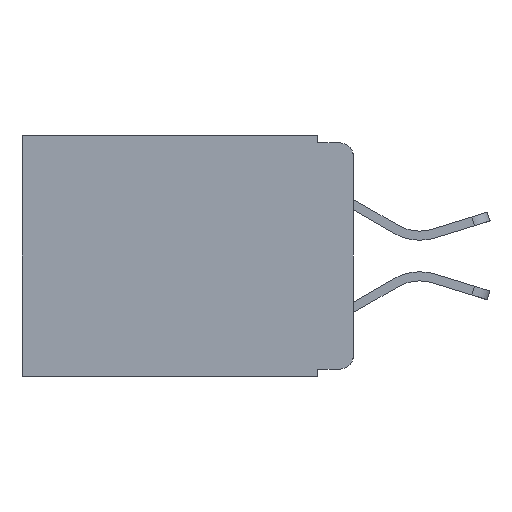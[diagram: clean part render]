
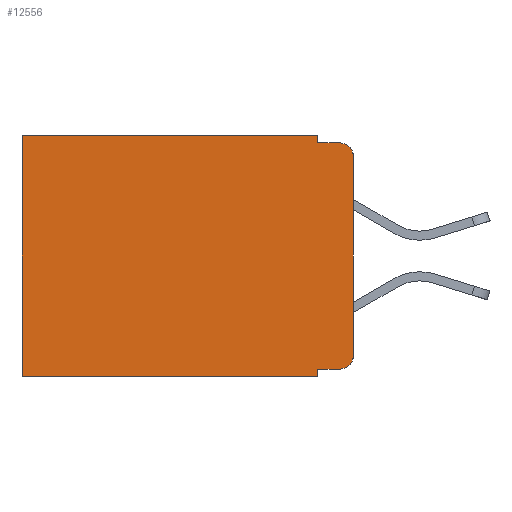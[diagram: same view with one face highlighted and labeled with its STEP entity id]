
A CAD part, left-side view. The second image highlights one B-rep face of the part: STEP entity #12556.
In plain terms, the highlighted planar face has unit normal (-1, 0, 0).
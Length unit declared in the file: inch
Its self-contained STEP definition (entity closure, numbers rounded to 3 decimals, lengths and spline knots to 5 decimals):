
#97 = EDGE_CURVE ( 'NONE', #14052, #8095, #5089, .T. ) ;
#119 = AXIS2_PLACEMENT_3D ( 'NONE', #12632, #4938, #13936 ) ;
#271 = CARTESIAN_POINT ( 'NONE',  ( 0.298, 0., 0. ) ) ;
#314 = CARTESIAN_POINT ( 'NONE',  ( 0.298, 0.051, -0.01 ) ) ;
#788 = ORIENTED_EDGE ( 'NONE', *, *, #12742, .T. ) ;
#1022 = CARTESIAN_POINT ( 'NONE',  ( 0.298, 0.02, -0.03 ) ) ;
#1136 = LINE ( 'NONE', #6046, #13415 ) ;
#1332 = CARTESIAN_POINT ( 'NONE',  ( 0.298, 0.051, 0. ) ) ;
#1670 = CARTESIAN_POINT ( 'NONE',  ( 0.298, 0.02, -0.333 ) ) ;
#1700 = FACE_OUTER_BOUND ( 'NONE', #5446, .T. ) ;
#1911 = VECTOR ( 'NONE', #9954, 39.37008 ) ;
#1912 = EDGE_CURVE ( 'NONE', #10570, #8095, #8886, .T. ) ;
#2055 = ORIENTED_EDGE ( 'NONE', *, *, #13623, .F. ) ;
#2117 = VERTEX_POINT ( 'NONE', #11443 ) ;
#2303 = VECTOR ( 'NONE', #10641, 39.37008 ) ;
#2398 = LINE ( 'NONE', #13743, #15792 ) ;
#2770 = VERTEX_POINT ( 'NONE', #1670 ) ;
#3006 = DIRECTION ( 'NONE',  ( 0., 0., -1. ) ) ;
#3040 = DIRECTION ( 'NONE',  ( -1., 0., 0. ) ) ;
#3200 = EDGE_CURVE ( 'NONE', #10178, #6726, #1136, .T. ) ;
#3749 = LINE ( 'NONE', #7935, #13255 ) ;
#4411 = CARTESIAN_POINT ( 'NONE',  ( 0.298, 0.051, -0.333 ) ) ;
#4774 = CIRCLE ( 'NONE', #119, 0.02 ) ;
#4907 = CARTESIAN_POINT ( 'NONE',  ( 0.298, 0.02, -0.01 ) ) ;
#4938 = DIRECTION ( 'NONE',  ( -1., 0., 0. ) ) ;
#4965 = VERTEX_POINT ( 'NONE', #5046 ) ;
#5046 = CARTESIAN_POINT ( 'NONE',  ( 0.298, 0., -0.313 ) ) ;
#5089 = LINE ( 'NONE', #314, #8149 ) ;
#5101 = CARTESIAN_POINT ( 'NONE',  ( 0.298, 0.051, -0.01 ) ) ;
#5204 = VECTOR ( 'NONE', #7310, 39.37008 ) ;
#5446 = EDGE_LOOP ( 'NONE', ( #7200, #6386, #6957, #6941, #7056, #12073, #5728, #2055, #788, #9640 ) ) ;
#5728 = ORIENTED_EDGE ( 'NONE', *, *, #10323, .F. ) ;
#5920 = LINE ( 'NONE', #6107, #1911 ) ;
#6046 = CARTESIAN_POINT ( 'NONE',  ( 0.298, 0., 0. ) ) ;
#6107 = CARTESIAN_POINT ( 'NONE',  ( 0.298, 0.051, -0.333 ) ) ;
#6386 = ORIENTED_EDGE ( 'NONE', *, *, #1912, .T. ) ;
#6726 = VERTEX_POINT ( 'NONE', #9935 ) ;
#6941 = ORIENTED_EDGE ( 'NONE', *, *, #16142, .F. ) ;
#6957 = ORIENTED_EDGE ( 'NONE', *, *, #97, .F. ) ;
#7056 = ORIENTED_EDGE ( 'NONE', *, *, #3200, .T. ) ;
#7086 = CARTESIAN_POINT ( 'NONE',  ( 0.298, 0.051, 0. ) ) ;
#7183 = VERTEX_POINT ( 'NONE', #4411 ) ;
#7200 = ORIENTED_EDGE ( 'NONE', *, *, #8176, .F. ) ;
#7310 = DIRECTION ( 'NONE',  ( 0., 0., -1. ) ) ;
#7895 = DIRECTION ( 'NONE',  ( 0., 0., -1. ) ) ;
#7935 = CARTESIAN_POINT ( 'NONE',  ( 0.298, 0., 0. ) ) ;
#8095 = VERTEX_POINT ( 'NONE', #4907 ) ;
#8149 = VECTOR ( 'NONE', #14157, 39.37008 ) ;
#8176 = EDGE_CURVE ( 'NONE', #10570, #4965, #3749, .T. ) ;
#8886 = CIRCLE ( 'NONE', #12116, 0.02 ) ;
#9151 = CARTESIAN_POINT ( 'NONE',  ( 0.298, 0., -0.03 ) ) ;
#9640 = ORIENTED_EDGE ( 'NONE', *, *, #11045, .T. ) ;
#9935 = CARTESIAN_POINT ( 'NONE',  ( 0.298, 0.473, 0. ) ) ;
#9942 = DIRECTION ( 'NONE',  ( 0., 1., 0. ) ) ;
#9954 = DIRECTION ( 'NONE',  ( 0., -1., 0. ) ) ;
#10178 = VERTEX_POINT ( 'NONE', #7086 ) ;
#10323 = EDGE_CURVE ( 'NONE', #2117, #10960, #2398, .T. ) ;
#10435 = DIRECTION ( 'NONE',  ( 0., 1., 0. ) ) ;
#10563 = DIRECTION ( 'NONE',  ( 0., 0., -1. ) ) ;
#10570 = VERTEX_POINT ( 'NONE', #9151 ) ;
#10641 = DIRECTION ( 'NONE',  ( 0., 0., -1. ) ) ;
#10832 = DIRECTION ( 'NONE',  ( 1., 0., 0. ) ) ;
#10960 = VERTEX_POINT ( 'NONE', #16233 ) ;
#11045 = EDGE_CURVE ( 'NONE', #2770, #4965, #4774, .T. ) ;
#11443 = CARTESIAN_POINT ( 'NONE',  ( 0.298, 0.051, -0.343 ) ) ;
#12073 = ORIENTED_EDGE ( 'NONE', *, *, #15301, .T. ) ;
#12116 = AXIS2_PLACEMENT_3D ( 'NONE', #1022, #3040, #7895 ) ;
#12366 = CARTESIAN_POINT ( 'NONE',  ( 0.298, 0.473, 0. ) ) ;
#12410 = LINE ( 'NONE', #1332, #13198 ) ;
#12556 = ADVANCED_FACE ( 'NONE', ( #1700 ), #15893, .F. ) ;
#12632 = CARTESIAN_POINT ( 'NONE',  ( 0.298, 0.02, -0.313 ) ) ;
#12742 = EDGE_CURVE ( 'NONE', #7183, #2770, #5920, .T. ) ;
#13109 = LINE ( 'NONE', #15754, #2303 ) ;
#13198 = VECTOR ( 'NONE', #10563, 39.37008 ) ;
#13255 = VECTOR ( 'NONE', #14290, 39.37008 ) ;
#13415 = VECTOR ( 'NONE', #10435, 39.37008 ) ;
#13623 = EDGE_CURVE ( 'NONE', #7183, #2117, #13109, .T. ) ;
#13743 = CARTESIAN_POINT ( 'NONE',  ( 0.298, 0., -0.343 ) ) ;
#13936 = DIRECTION ( 'NONE',  ( 0., 0., -1. ) ) ;
#14052 = VERTEX_POINT ( 'NONE', #5101 ) ;
#14157 = DIRECTION ( 'NONE',  ( 0., -1., 0. ) ) ;
#14290 = DIRECTION ( 'NONE',  ( 0., 0., -1. ) ) ;
#15031 = LINE ( 'NONE', #12366, #5204 ) ;
#15131 = AXIS2_PLACEMENT_3D ( 'NONE', #271, #10832, #3006 ) ;
#15301 = EDGE_CURVE ( 'NONE', #6726, #10960, #15031, .T. ) ;
#15754 = CARTESIAN_POINT ( 'NONE',  ( 0.298, 0.051, 0. ) ) ;
#15792 = VECTOR ( 'NONE', #9942, 39.37008 ) ;
#15893 = PLANE ( 'NONE',  #15131 ) ;
#16142 = EDGE_CURVE ( 'NONE', #10178, #14052, #12410, .T. ) ;
#16233 = CARTESIAN_POINT ( 'NONE',  ( 0.298, 0.473, -0.343 ) ) ;
